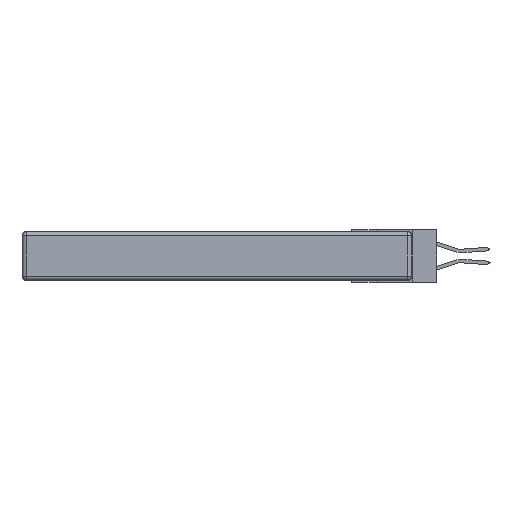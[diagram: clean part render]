
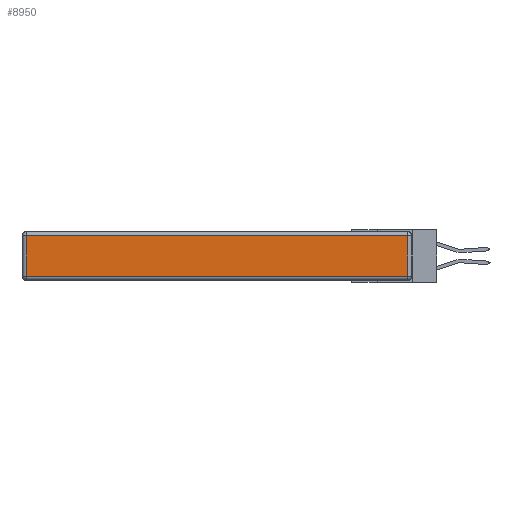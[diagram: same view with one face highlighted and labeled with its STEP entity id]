
A CAD part, left-side view. The second image highlights one B-rep face of the part: STEP entity #8950.
In plain terms, the highlighted planar face has unit normal (-1, 0, 0).
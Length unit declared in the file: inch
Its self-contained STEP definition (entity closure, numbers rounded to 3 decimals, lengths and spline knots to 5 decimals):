
#363 = CARTESIAN_POINT ( 'NONE',  ( 0., 2.72, -0.313 ) ) ;
#948 = ORIENTED_EDGE ( 'NONE', *, *, #32502, .T. ) ;
#1003 = VECTOR ( 'NONE', #14188, 39.37008 ) ;
#1694 = EDGE_CURVE ( 'NONE', #22515, #35494, #27648, .T. ) ;
#1875 = ORIENTED_EDGE ( 'NONE', *, *, #32592, .T. ) ;
#2461 = DIRECTION ( 'NONE',  ( 0., 0., -1. ) ) ;
#3088 = FACE_OUTER_BOUND ( 'NONE', #20477, .T. ) ;
#3517 = AXIS2_PLACEMENT_3D ( 'NONE', #34913, #10276, #21567 ) ;
#3643 = LINE ( 'NONE', #17196, #5376 ) ;
#5376 = VECTOR ( 'NONE', #25475, 39.37008 ) ;
#8950 = ADVANCED_FACE ( 'NONE', ( #3088 ), #32526, .T. ) ;
#10276 = DIRECTION ( 'NONE',  ( -1., 0., 0. ) ) ;
#14087 = VERTEX_POINT ( 'NONE', #363 ) ;
#14188 = DIRECTION ( 'NONE',  ( 0., 0., 1. ) ) ;
#16062 = VECTOR ( 'NONE', #29198, 39.37008 ) ;
#16112 = ORIENTED_EDGE ( 'NONE', *, *, #1694, .T. ) ;
#17196 = CARTESIAN_POINT ( 'NONE',  ( 0., 0., -0.313 ) ) ;
#19715 = CARTESIAN_POINT ( 'NONE',  ( 0., 0.03, -0.03 ) ) ;
#20477 = EDGE_LOOP ( 'NONE', ( #948, #16112, #1875, #33539 ) ) ;
#21567 = DIRECTION ( 'NONE',  ( 0., 0., 1. ) ) ;
#22515 = VERTEX_POINT ( 'NONE', #32279 ) ;
#22693 = CARTESIAN_POINT ( 'NONE',  ( 0., 0.03, -0.343 ) ) ;
#22986 = VECTOR ( 'NONE', #2461, 39.37008 ) ;
#24243 = CARTESIAN_POINT ( 'NONE',  ( 0., 2.72, -0.03 ) ) ;
#25197 = VERTEX_POINT ( 'NONE', #24243 ) ;
#25475 = DIRECTION ( 'NONE',  ( 0., -1., 0. ) ) ;
#25935 = LINE ( 'NONE', #26179, #16062 ) ;
#26179 = CARTESIAN_POINT ( 'NONE',  ( 0., 2.75, -0.03 ) ) ;
#27648 = LINE ( 'NONE', #22693, #1003 ) ;
#29198 = DIRECTION ( 'NONE',  ( 0., 1., 0. ) ) ;
#29874 = EDGE_CURVE ( 'NONE', #25197, #14087, #29964, .T. ) ;
#29964 = LINE ( 'NONE', #32707, #22986 ) ;
#32279 = CARTESIAN_POINT ( 'NONE',  ( 0., 0.03, -0.313 ) ) ;
#32502 = EDGE_CURVE ( 'NONE', #14087, #22515, #3643, .T. ) ;
#32526 = PLANE ( 'NONE',  #3517 ) ;
#32592 = EDGE_CURVE ( 'NONE', #35494, #25197, #25935, .T. ) ;
#32707 = CARTESIAN_POINT ( 'NONE',  ( 0., 2.72, -0.343 ) ) ;
#33539 = ORIENTED_EDGE ( 'NONE', *, *, #29874, .T. ) ;
#34913 = CARTESIAN_POINT ( 'NONE',  ( 0., 0., -0.343 ) ) ;
#35494 = VERTEX_POINT ( 'NONE', #19715 ) ;
